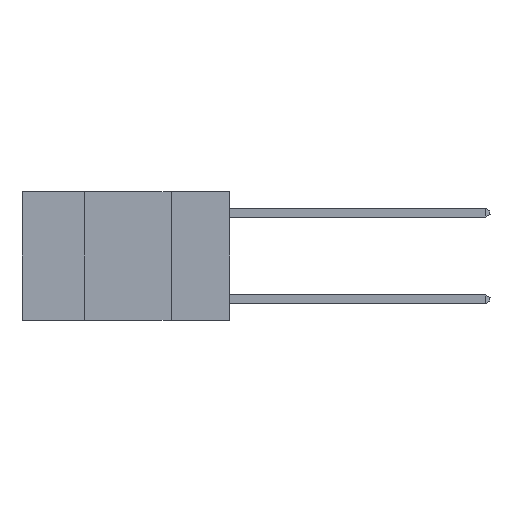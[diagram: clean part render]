
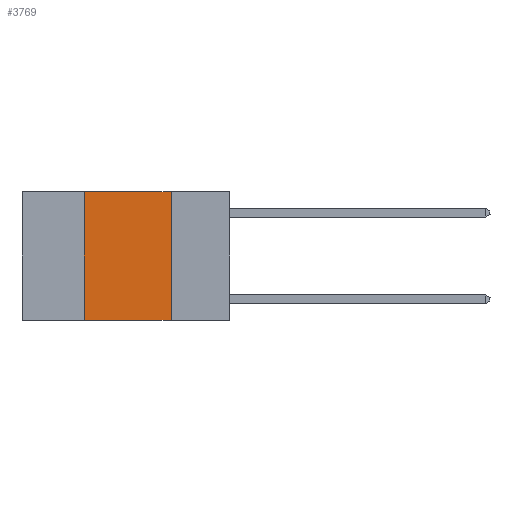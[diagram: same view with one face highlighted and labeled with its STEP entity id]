
A CAD part, left-side view. The second image highlights one B-rep face of the part: STEP entity #3769.
In plain terms, the highlighted planar face has unit normal (-1, 0, 0).
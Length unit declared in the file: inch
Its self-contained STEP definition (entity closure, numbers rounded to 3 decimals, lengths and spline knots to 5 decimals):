
#586 = LINE ( 'NONE', #6524, #7338 ) ;
#924 = DIRECTION ( 'NONE',  ( 0., 0., 1. ) ) ;
#1105 = VECTOR ( 'NONE', #10501, 39.37008 ) ;
#1357 = DIRECTION ( 'NONE',  ( 1., 0., 0. ) ) ;
#1892 = EDGE_LOOP ( 'NONE', ( #6059, #4881, #2336, #2208 ) ) ;
#2174 = DIRECTION ( 'NONE',  ( 0., -1., 0. ) ) ;
#2208 = ORIENTED_EDGE ( 'NONE', *, *, #10297, .T. ) ;
#2296 = AXIS2_PLACEMENT_3D ( 'NONE', #2571, #1357, #12406 ) ;
#2336 = ORIENTED_EDGE ( 'NONE', *, *, #5779, .F. ) ;
#2571 = CARTESIAN_POINT ( 'NONE',  ( 0., 0.6, 0. ) ) ;
#3769 = ADVANCED_FACE ( 'NONE', ( #9889 ), #7547, .F. ) ;
#4633 = CARTESIAN_POINT ( 'NONE',  ( 0., 0.17, -0.37 ) ) ;
#4881 = ORIENTED_EDGE ( 'NONE', *, *, #7312, .F. ) ;
#4896 = VERTEX_POINT ( 'NONE', #10679 ) ;
#5480 = DIRECTION ( 'NONE',  ( 0., -1., 0. ) ) ;
#5779 = EDGE_CURVE ( 'NONE', #12183, #4896, #13084, .T. ) ;
#6059 = ORIENTED_EDGE ( 'NONE', *, *, #13277, .F. ) ;
#6524 = CARTESIAN_POINT ( 'NONE',  ( 0., 0.6, 0. ) ) ;
#6657 = VERTEX_POINT ( 'NONE', #4633 ) ;
#6863 = CARTESIAN_POINT ( 'NONE',  ( 0., 0.42, 0. ) ) ;
#7021 = VERTEX_POINT ( 'NONE', #15750 ) ;
#7312 = EDGE_CURVE ( 'NONE', #4896, #7021, #586, .T. ) ;
#7338 = VECTOR ( 'NONE', #5480, 39.37008 ) ;
#7547 = PLANE ( 'NONE',  #2296 ) ;
#8204 = CARTESIAN_POINT ( 'NONE',  ( 0., 0.6, -0.37 ) ) ;
#8706 = VECTOR ( 'NONE', #2174, 39.37008 ) ;
#9889 = FACE_OUTER_BOUND ( 'NONE', #1892, .T. ) ;
#10297 = EDGE_CURVE ( 'NONE', #12183, #6657, #14275, .T. ) ;
#10427 = LINE ( 'NONE', #12518, #1105 ) ;
#10501 = DIRECTION ( 'NONE',  ( 0., 0., -1. ) ) ;
#10679 = CARTESIAN_POINT ( 'NONE',  ( 0., 0.42, 0. ) ) ;
#11115 = CARTESIAN_POINT ( 'NONE',  ( 0., 0.42, -0.37 ) ) ;
#11692 = VECTOR ( 'NONE', #924, 39.37008 ) ;
#12183 = VERTEX_POINT ( 'NONE', #11115 ) ;
#12406 = DIRECTION ( 'NONE',  ( 0., 0., -1. ) ) ;
#12518 = CARTESIAN_POINT ( 'NONE',  ( 0., 0.17, 0. ) ) ;
#13084 = LINE ( 'NONE', #6863, #11692 ) ;
#13277 = EDGE_CURVE ( 'NONE', #7021, #6657, #10427, .T. ) ;
#14275 = LINE ( 'NONE', #8204, #8706 ) ;
#15750 = CARTESIAN_POINT ( 'NONE',  ( 0., 0.17, 0. ) ) ;
